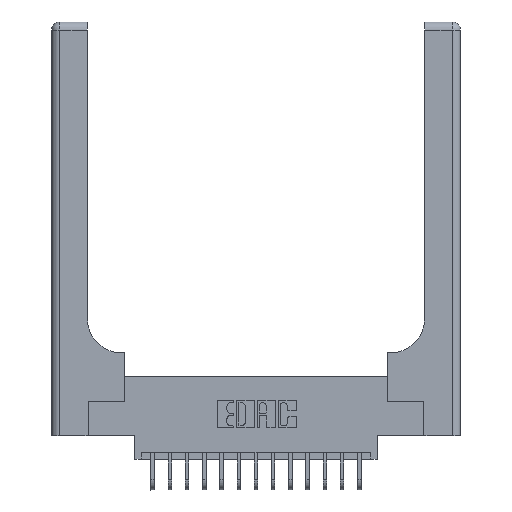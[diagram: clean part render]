
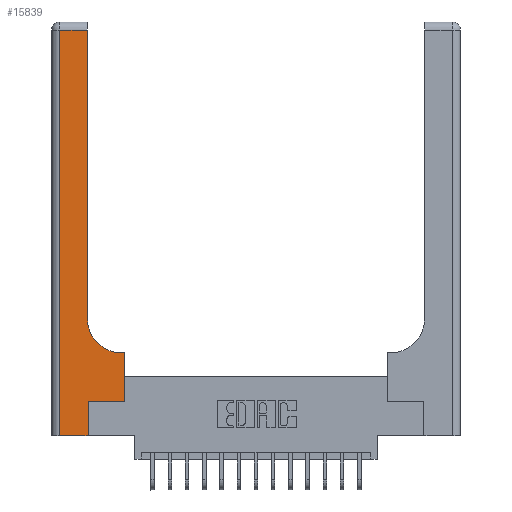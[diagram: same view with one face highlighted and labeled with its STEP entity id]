
A CAD part, top view. The second image highlights one B-rep face of the part: STEP entity #15839.
In plain terms, the highlighted planar face has unit normal (0, 0, 1).
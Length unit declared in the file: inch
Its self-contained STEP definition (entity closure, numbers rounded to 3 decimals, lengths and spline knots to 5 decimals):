
#46 = DIRECTION ( 'NONE',  ( 0., 1., 0. ) ) ;
#68 = ORIENTED_EDGE ( 'NONE', *, *, #3723, .T. ) ;
#236 = VERTEX_POINT ( 'NONE', #4620 ) ;
#1661 = ORIENTED_EDGE ( 'NONE', *, *, #8624, .T. ) ;
#2663 = EDGE_LOOP ( 'NONE', ( #10169, #1661, #13646, #14784, #68, #6914, #15128, #3978, #8524 ) ) ;
#3164 = EDGE_CURVE ( 'NONE', #6209, #18995, #8022, .T. ) ;
#3351 = EDGE_CURVE ( 'NONE', #236, #15717, #11528, .T. ) ;
#3434 = VERTEX_POINT ( 'NONE', #18110 ) ;
#3514 = CARTESIAN_POINT ( 'NONE',  ( 0., 2.94, 0.37 ) ) ;
#3723 = EDGE_CURVE ( 'NONE', #15717, #14704, #17476, .T. ) ;
#3978 = ORIENTED_EDGE ( 'NONE', *, *, #11073, .T. ) ;
#4059 = PLANE ( 'NONE',  #16801 ) ;
#4184 = CIRCLE ( 'NONE', #16731, 0.25 ) ;
#4361 = LINE ( 'NONE', #16564, #4507 ) ;
#4507 = VECTOR ( 'NONE', #19888, 39.37008 ) ;
#4620 = CARTESIAN_POINT ( 'NONE',  ( 0.06, 0., 0.37 ) ) ;
#4672 = DIRECTION ( 'NONE',  ( 0., -1., 0. ) ) ;
#4734 = CARTESIAN_POINT ( 'NONE',  ( 0.26, 2.94, 0.37 ) ) ;
#4914 = EDGE_CURVE ( 'NONE', #7581, #12626, #7707, .T. ) ;
#5287 = DIRECTION ( 'NONE',  ( 0., 1., 0. ) ) ;
#6209 = VERTEX_POINT ( 'NONE', #19304 ) ;
#6446 = EDGE_CURVE ( 'NONE', #16918, #236, #17163, .T. ) ;
#6746 = VECTOR ( 'NONE', #8063, 39.37008 ) ;
#6914 = ORIENTED_EDGE ( 'NONE', *, *, #13052, .T. ) ;
#7423 = DIRECTION ( 'NONE',  ( 1., 0., 0. ) ) ;
#7495 = CARTESIAN_POINT ( 'NONE',  ( 0.528, 0.25, 0.37 ) ) ;
#7581 = VERTEX_POINT ( 'NONE', #7495 ) ;
#7707 = LINE ( 'NONE', #13848, #17572 ) ;
#8022 = LINE ( 'NONE', #9827, #9491 ) ;
#8063 = DIRECTION ( 'NONE',  ( -1., 0., 0. ) ) ;
#8350 = LINE ( 'NONE', #3514, #9582 ) ;
#8524 = ORIENTED_EDGE ( 'NONE', *, *, #11613, .T. ) ;
#8526 = CARTESIAN_POINT ( 'NONE',  ( 0., 0., 0.37 ) ) ;
#8624 = EDGE_CURVE ( 'NONE', #18995, #16918, #8350, .T. ) ;
#8923 = CARTESIAN_POINT ( 'NONE',  ( 0.528, 0.6, 0.37 ) ) ;
#9373 = CARTESIAN_POINT ( 'NONE',  ( 0.26, 0.6, 0.37 ) ) ;
#9491 = VECTOR ( 'NONE', #18820, 39.37008 ) ;
#9501 = CARTESIAN_POINT ( 'NONE',  ( 0.06, 3., 0.37 ) ) ;
#9582 = VECTOR ( 'NONE', #11165, 39.37008 ) ;
#9827 = CARTESIAN_POINT ( 'NONE',  ( 0.26, 3., 0.37 ) ) ;
#10169 = ORIENTED_EDGE ( 'NONE', *, *, #3164, .T. ) ;
#10203 = DIRECTION ( 'NONE',  ( 0., 0., -1. ) ) ;
#10641 = VECTOR ( 'NONE', #4672, 39.37008 ) ;
#11073 = EDGE_CURVE ( 'NONE', #12626, #3434, #18560, .T. ) ;
#11165 = DIRECTION ( 'NONE',  ( -1., 0., 0. ) ) ;
#11528 = LINE ( 'NONE', #8526, #11746 ) ;
#11601 = FACE_OUTER_BOUND ( 'NONE', #2663, .T. ) ;
#11613 = EDGE_CURVE ( 'NONE', #3434, #6209, #4184, .T. ) ;
#11746 = VECTOR ( 'NONE', #19118, 39.37008 ) ;
#12626 = VERTEX_POINT ( 'NONE', #8923 ) ;
#13052 = EDGE_CURVE ( 'NONE', #14704, #7581, #4361, .T. ) ;
#13114 = CARTESIAN_POINT ( 'NONE',  ( 0., 3., 0.37 ) ) ;
#13327 = CARTESIAN_POINT ( 'NONE',  ( 0.265, 0., 0.37 ) ) ;
#13506 = CARTESIAN_POINT ( 'NONE',  ( 0.265, 0.25, 0.37 ) ) ;
#13545 = VECTOR ( 'NONE', #5287, 39.37008 ) ;
#13646 = ORIENTED_EDGE ( 'NONE', *, *, #6446, .T. ) ;
#13848 = CARTESIAN_POINT ( 'NONE',  ( 0.528, 0.25, 0.37 ) ) ;
#14329 = CARTESIAN_POINT ( 'NONE',  ( 0.265, 0., 0.37 ) ) ;
#14704 = VERTEX_POINT ( 'NONE', #13506 ) ;
#14784 = ORIENTED_EDGE ( 'NONE', *, *, #3351, .T. ) ;
#15128 = ORIENTED_EDGE ( 'NONE', *, *, #4914, .T. ) ;
#15179 = DIRECTION ( 'NONE',  ( 0., 0., -1. ) ) ;
#15717 = VERTEX_POINT ( 'NONE', #14329 ) ;
#15749 = CARTESIAN_POINT ( 'NONE',  ( 0.06, 2.94, 0.37 ) ) ;
#15839 = ADVANCED_FACE ( 'NONE', ( #11601 ), #4059, .F. ) ;
#16564 = CARTESIAN_POINT ( 'NONE',  ( 0.265, 0.25, 0.37 ) ) ;
#16731 = AXIS2_PLACEMENT_3D ( 'NONE', #19632, #15179, #7423 ) ;
#16801 = AXIS2_PLACEMENT_3D ( 'NONE', #13114, #10203, #17784 ) ;
#16918 = VERTEX_POINT ( 'NONE', #15749 ) ;
#17163 = LINE ( 'NONE', #9501, #10641 ) ;
#17476 = LINE ( 'NONE', #13327, #13545 ) ;
#17572 = VECTOR ( 'NONE', #46, 39.37008 ) ;
#17784 = DIRECTION ( 'NONE',  ( -1., 0., 0. ) ) ;
#18110 = CARTESIAN_POINT ( 'NONE',  ( 0.51, 0.6, 0.37 ) ) ;
#18560 = LINE ( 'NONE', #9373, #6746 ) ;
#18820 = DIRECTION ( 'NONE',  ( 0., 1., 0. ) ) ;
#18995 = VERTEX_POINT ( 'NONE', #4734 ) ;
#19118 = DIRECTION ( 'NONE',  ( 1., 0., 0. ) ) ;
#19304 = CARTESIAN_POINT ( 'NONE',  ( 0.26, 0.85, 0.37 ) ) ;
#19632 = CARTESIAN_POINT ( 'NONE',  ( 0.51, 0.85, 0.37 ) ) ;
#19888 = DIRECTION ( 'NONE',  ( 1., 0., 0. ) ) ;
